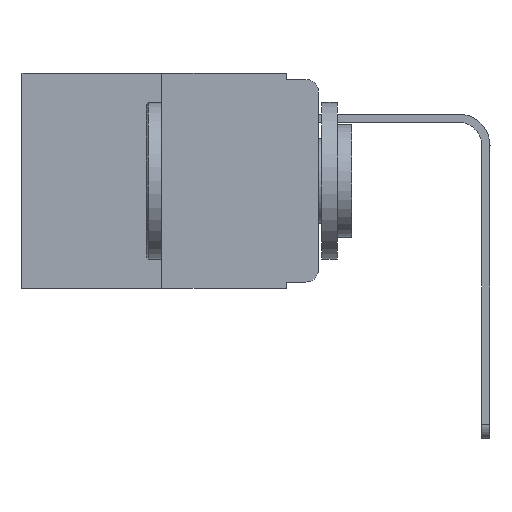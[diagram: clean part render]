
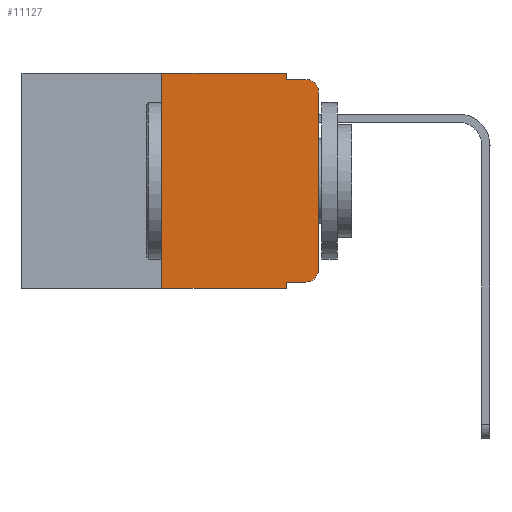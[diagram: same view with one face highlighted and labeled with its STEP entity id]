
A CAD part, left-side view. The second image highlights one B-rep face of the part: STEP entity #11127.
In plain terms, the highlighted planar face has unit normal (-1, 0, 0).
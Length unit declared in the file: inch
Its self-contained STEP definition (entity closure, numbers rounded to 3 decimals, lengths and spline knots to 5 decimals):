
#146 = ORIENTED_EDGE ( 'NONE', *, *, #1241, .T. ) ;
#292 = VECTOR ( 'NONE', #399, 39.37008 ) ;
#353 = DIRECTION ( 'NONE',  ( 1., 0., 0. ) ) ;
#397 = VECTOR ( 'NONE', #2542, 39.37008 ) ;
#399 = DIRECTION ( 'NONE',  ( 0., -1., 0. ) ) ;
#612 = VERTEX_POINT ( 'NONE', #17742 ) ;
#1062 = VERTEX_POINT ( 'NONE', #1551 ) ;
#1241 = EDGE_CURVE ( 'NONE', #4178, #14104, #6806, .T. ) ;
#1407 = CARTESIAN_POINT ( 'NONE',  ( 0., 0.051, 0. ) ) ;
#1427 = DIRECTION ( 'NONE',  ( 0., 0., 1. ) ) ;
#1541 = LINE ( 'NONE', #10699, #2662 ) ;
#1551 = CARTESIAN_POINT ( 'NONE',  ( 0., 0.051, 0. ) ) ;
#1734 = EDGE_CURVE ( 'NONE', #12724, #14104, #12500, .T. ) ;
#2370 = ORIENTED_EDGE ( 'NONE', *, *, #9720, .F. ) ;
#2542 = DIRECTION ( 'NONE',  ( 0., -1., 0. ) ) ;
#2662 = VECTOR ( 'NONE', #9317, 39.37008 ) ;
#2713 = DIRECTION ( 'NONE',  ( 0., 0., -1. ) ) ;
#2914 = VERTEX_POINT ( 'NONE', #9629 ) ;
#2935 = EDGE_CURVE ( 'NONE', #2914, #17958, #12664, .T. ) ;
#3141 = CARTESIAN_POINT ( 'NONE',  ( 0., 0.051, -0.01 ) ) ;
#3169 = DIRECTION ( 'NONE',  ( 0., 0., -1. ) ) ;
#3581 = EDGE_CURVE ( 'NONE', #17958, #13285, #17434, .T. ) ;
#4178 = VERTEX_POINT ( 'NONE', #6804 ) ;
#4258 = ORIENTED_EDGE ( 'NONE', *, *, #11357, .T. ) ;
#4318 = VERTEX_POINT ( 'NONE', #12870 ) ;
#4742 = AXIS2_PLACEMENT_3D ( 'NONE', #6073, #353, #3169 ) ;
#5183 = VECTOR ( 'NONE', #16220, 39.37008 ) ;
#5283 = ORIENTED_EDGE ( 'NONE', *, *, #2935, .T. ) ;
#5682 = DIRECTION ( 'NONE',  ( 0., 0., -1. ) ) ;
#6073 = CARTESIAN_POINT ( 'NONE',  ( 0., 0.473, 0. ) ) ;
#6519 = LINE ( 'NONE', #14283, #17712 ) ;
#6647 = EDGE_CURVE ( 'NONE', #13285, #4178, #17253, .T. ) ;
#6763 = EDGE_CURVE ( 'NONE', #15262, #612, #13870, .T. ) ;
#6804 = CARTESIAN_POINT ( 'NONE',  ( 0., 0., -0.03 ) ) ;
#6806 = CIRCLE ( 'NONE', #15239, 0.02 ) ;
#6929 = VECTOR ( 'NONE', #1427, 39.37008 ) ;
#7030 = DIRECTION ( 'NONE',  ( -1., 0., 0. ) ) ;
#7093 = CARTESIAN_POINT ( 'NONE',  ( 0., 0.02, -0.03 ) ) ;
#7238 = ORIENTED_EDGE ( 'NONE', *, *, #3581, .T. ) ;
#7267 = CARTESIAN_POINT ( 'NONE',  ( 0., 0., 0. ) ) ;
#7693 = CARTESIAN_POINT ( 'NONE',  ( 0., 0.25, -0.343 ) ) ;
#7736 = VECTOR ( 'NONE', #11951, 39.37008 ) ;
#8037 = ORIENTED_EDGE ( 'NONE', *, *, #1734, .F. ) ;
#9056 = PLANE ( 'NONE',  #4742 ) ;
#9090 = AXIS2_PLACEMENT_3D ( 'NONE', #12760, #7030, #2713 ) ;
#9096 = CARTESIAN_POINT ( 'NONE',  ( 0., 0., -0.313 ) ) ;
#9317 = DIRECTION ( 'NONE',  ( 0., -1., 0. ) ) ;
#9629 = CARTESIAN_POINT ( 'NONE',  ( 0., 0.051, -0.333 ) ) ;
#9720 = EDGE_CURVE ( 'NONE', #1062, #12724, #17423, .T. ) ;
#9770 = DIRECTION ( 'NONE',  ( 0., 0., -1. ) ) ;
#10509 = LINE ( 'NONE', #11967, #292 ) ;
#10699 = CARTESIAN_POINT ( 'NONE',  ( 0., 0.473, 0. ) ) ;
#11127 = ADVANCED_FACE ( 'NONE', ( #16425 ), #9056, .F. ) ;
#11305 = DIRECTION ( 'NONE',  ( -1., 0., 0. ) ) ;
#11357 = EDGE_CURVE ( 'NONE', #15262, #4318, #10509, .T. ) ;
#11901 = ORIENTED_EDGE ( 'NONE', *, *, #18098, .F. ) ;
#11951 = DIRECTION ( 'NONE',  ( 0., -1., 0. ) ) ;
#11967 = CARTESIAN_POINT ( 'NONE',  ( 0., 0.473, -0.343 ) ) ;
#12441 = CARTESIAN_POINT ( 'NONE',  ( 0., 0.02, -0.333 ) ) ;
#12500 = LINE ( 'NONE', #3141, #7736 ) ;
#12664 = LINE ( 'NONE', #18775, #397 ) ;
#12724 = VERTEX_POINT ( 'NONE', #17946 ) ;
#12760 = CARTESIAN_POINT ( 'NONE',  ( 0., 0.02, -0.313 ) ) ;
#12870 = CARTESIAN_POINT ( 'NONE',  ( 0., 0.051, -0.343 ) ) ;
#13030 = EDGE_LOOP ( 'NONE', ( #17348, #146, #8037, #2370, #16330, #16461, #4258, #11901, #5283, #7238 ) ) ;
#13285 = VERTEX_POINT ( 'NONE', #9096 ) ;
#13870 = LINE ( 'NONE', #14709, #5183 ) ;
#14104 = VERTEX_POINT ( 'NONE', #16870 ) ;
#14283 = CARTESIAN_POINT ( 'NONE',  ( 0., 0.051, 0. ) ) ;
#14360 = DIRECTION ( 'NONE',  ( 0., 0., -1. ) ) ;
#14709 = CARTESIAN_POINT ( 'NONE',  ( 0., 0.25, 0. ) ) ;
#15111 = VECTOR ( 'NONE', #5682, 39.37008 ) ;
#15239 = AXIS2_PLACEMENT_3D ( 'NONE', #7093, #11305, #14360 ) ;
#15262 = VERTEX_POINT ( 'NONE', #7693 ) ;
#16220 = DIRECTION ( 'NONE',  ( 0., 0., 1. ) ) ;
#16330 = ORIENTED_EDGE ( 'NONE', *, *, #18522, .F. ) ;
#16425 = FACE_OUTER_BOUND ( 'NONE', #13030, .T. ) ;
#16461 = ORIENTED_EDGE ( 'NONE', *, *, #6763, .F. ) ;
#16870 = CARTESIAN_POINT ( 'NONE',  ( 0., 0.02, -0.01 ) ) ;
#17253 = LINE ( 'NONE', #7267, #6929 ) ;
#17348 = ORIENTED_EDGE ( 'NONE', *, *, #6647, .T. ) ;
#17423 = LINE ( 'NONE', #1407, #15111 ) ;
#17434 = CIRCLE ( 'NONE', #9090, 0.02 ) ;
#17712 = VECTOR ( 'NONE', #9770, 39.37008 ) ;
#17742 = CARTESIAN_POINT ( 'NONE',  ( 0., 0.25, 0. ) ) ;
#17946 = CARTESIAN_POINT ( 'NONE',  ( 0., 0.051, -0.01 ) ) ;
#17958 = VERTEX_POINT ( 'NONE', #12441 ) ;
#18098 = EDGE_CURVE ( 'NONE', #2914, #4318, #6519, .T. ) ;
#18522 = EDGE_CURVE ( 'NONE', #612, #1062, #1541, .T. ) ;
#18775 = CARTESIAN_POINT ( 'NONE',  ( 0., 0.051, -0.333 ) ) ;
